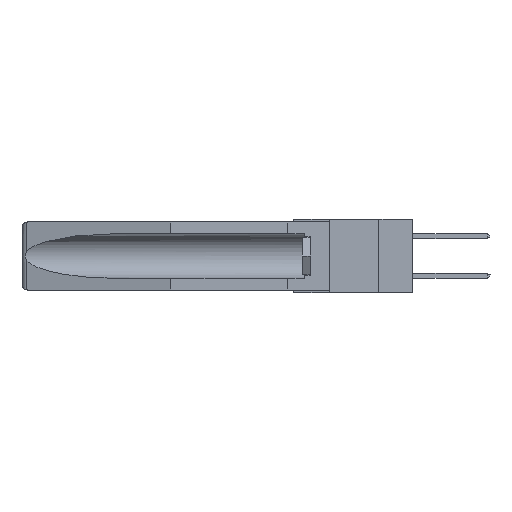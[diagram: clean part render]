
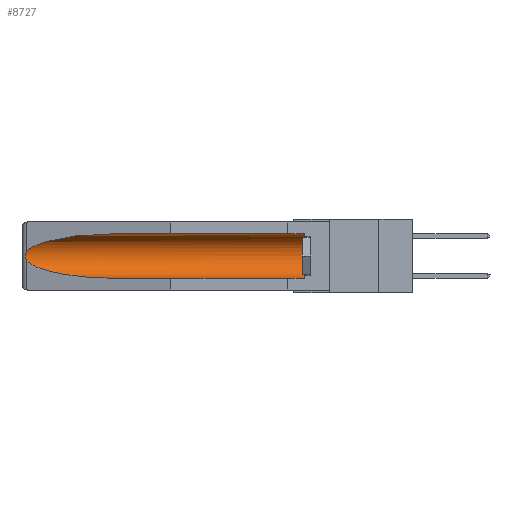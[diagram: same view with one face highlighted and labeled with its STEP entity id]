
A CAD part, left-side view. The second image highlights one B-rep face of the part: STEP entity #8727.
In plain terms, the highlighted cylindrical face has radius 2.857 mm (diameter 5.715 mm), a partial arc.
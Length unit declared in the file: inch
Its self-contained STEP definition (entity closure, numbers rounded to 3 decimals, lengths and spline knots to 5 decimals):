
#3 =( BOUNDED_CURVE ( )  B_SPLINE_CURVE ( 3, ( #23442, #5948, #15624, #5867 ),
 .UNSPECIFIED., .F., .F. ) 
 B_SPLINE_CURVE_WITH_KNOTS ( ( 4, 4 ),
 ( 0.1948, 1.5708 ),
 .UNSPECIFIED. ) 
 CURVE ( )  GEOMETRIC_REPRESENTATION_ITEM ( )  RATIONAL_B_SPLINE_CURVE ( ( 1., 0.848, 0.848, 1. ) ) 
 REPRESENTATION_ITEM ( '' )  );
#328 = EDGE_CURVE ( 'NONE', #17743, #17272, #1385, .T. ) ;
#438 = LINE ( 'NONE', #19097, #12175 ) ;
#829 = VERTEX_POINT ( 'NONE', #1903 ) ;
#1095 = ORIENTED_EDGE ( 'NONE', *, *, #6823, .T. ) ;
#1385 = B_SPLINE_CURVE_WITH_KNOTS ( 'NONE', 3,
 ( #20605, #16587, #24638, #8852, #22409, #8941, #18413, #16749, #18651, #12716 ),
 .UNSPECIFIED., .F., .F.,
 ( 4, 2, 2, 2, 4 ),
 ( 0., 0.00029, 0.00058, 0.00087, 0.00117 ),
 .UNSPECIFIED. ) ;
#1903 = CARTESIAN_POINT ( 'NONE',  ( 0.155, 0.126, -0.059 ) ) ;
#2323 = ORIENTED_EDGE ( 'NONE', *, *, #14738, .T. ) ;
#3191 = LINE ( 'NONE', #23447, #12203 ) ;
#3434 = CARTESIAN_POINT ( 'NONE',  ( 0.155, -0.30754, -0.1715 ) ) ;
#3540 = EDGE_CURVE ( 'NONE', #17736, #11007, #3191, .T. ) ;
#4085 = CARTESIAN_POINT ( 'NONE',  ( 0.155, 1.07973, -0.284 ) ) ;
#4556 = VERTEX_POINT ( 'NONE', #12770 ) ;
#4819 = CARTESIAN_POINT ( 'NONE',  ( 0.26537, 1.52718, -0.14972 ) ) ;
#4895 = CARTESIAN_POINT ( 'NONE',  ( 0.155, 1.07973, -0.059 ) ) ;
#5078 = DIRECTION ( 'NONE',  ( 0., 1., 0. ) ) ;
#5425 = DIRECTION ( 'NONE',  ( 0., -1., 0. ) ) ;
#5719 = ORIENTED_EDGE ( 'NONE', *, *, #24822, .T. ) ;
#5867 = CARTESIAN_POINT ( 'NONE',  ( 0.155, 1.07973, -0.284 ) ) ;
#5948 = CARTESIAN_POINT ( 'NONE',  ( 0.25451, 1.48313, -0.24835 ) ) ;
#6102 = CARTESIAN_POINT ( 'NONE',  ( 0.26537, 1.52718, -0.19328 ) ) ;
#6205 = FACE_OUTER_BOUND ( 'NONE', #23884, .T. ) ;
#6723 = CARTESIAN_POINT ( 'NONE',  ( 0.21114, 1.30732, -0.059 ) ) ;
#6823 = EDGE_CURVE ( 'NONE', #829, #4556, #438, .T. ) ;
#7104 = DIRECTION ( 'NONE',  ( 0., 0., 1. ) ) ;
#7859 = CARTESIAN_POINT ( 'NONE',  ( 0.26537, 1.52718, -0.14972 ) ) ;
#8727 = ADVANCED_FACE ( 'NONE', ( #6205 ), #10832, .F. ) ;
#8728 = CARTESIAN_POINT ( 'NONE',  ( 0.25451, 1.48313, -0.09465 ) ) ;
#8852 = CARTESIAN_POINT ( 'NONE',  ( 0.2673, 1.5327, -0.16383 ) ) ;
#8941 = CARTESIAN_POINT ( 'NONE',  ( 0.2675, 1.53308, -0.17534 ) ) ;
#9845 = AXIS2_PLACEMENT_3D ( 'NONE', #3434, #5078, #7104 ) ;
#10832 = CYLINDRICAL_SURFACE ( 'NONE', #9845, 0.1125 ) ;
#11007 = VERTEX_POINT ( 'NONE', #4085 ) ;
#12175 = VECTOR ( 'NONE', #13164, 39.37008 ) ;
#12203 = VECTOR ( 'NONE', #19569, 39.37008 ) ;
#12716 = CARTESIAN_POINT ( 'NONE',  ( 0.26537, 1.52718, -0.19328 ) ) ;
#12770 = CARTESIAN_POINT ( 'NONE',  ( 0.155, 1.07973, -0.059 ) ) ;
#13164 = DIRECTION ( 'NONE',  ( 0., 1., 0. ) ) ;
#13293 = DIRECTION ( 'NONE',  ( 0., 0., 1. ) ) ;
#13857 = ORIENTED_EDGE ( 'NONE', *, *, #23573, .T. ) ;
#14738 = EDGE_CURVE ( 'NONE', #17736, #829, #19754, .T. ) ;
#15480 = ORIENTED_EDGE ( 'NONE', *, *, #3540, .F. ) ;
#15624 = CARTESIAN_POINT ( 'NONE',  ( 0.21114, 1.30732, -0.284 ) ) ;
#16587 = CARTESIAN_POINT ( 'NONE',  ( 0.26597, 1.52961, -0.15275 ) ) ;
#16749 = CARTESIAN_POINT ( 'NONE',  ( 0.26655, 1.53094, -0.18657 ) ) ;
#17272 = VERTEX_POINT ( 'NONE', #6102 ) ;
#17665 = ORIENTED_EDGE ( 'NONE', *, *, #328, .T. ) ;
#17736 = VERTEX_POINT ( 'NONE', #25470 ) ;
#17743 = VERTEX_POINT ( 'NONE', #7859 ) ;
#18413 = CARTESIAN_POINT ( 'NONE',  ( 0.2673, 1.53269, -0.17917 ) ) ;
#18651 = CARTESIAN_POINT ( 'NONE',  ( 0.26597, 1.5296, -0.19026 ) ) ;
#19097 = CARTESIAN_POINT ( 'NONE',  ( 0.155, -0.30754, -0.059 ) ) ;
#19482 = AXIS2_PLACEMENT_3D ( 'NONE', #25062, #5425, #13293 ) ;
#19569 = DIRECTION ( 'NONE',  ( 0., 1., 0. ) ) ;
#19754 = CIRCLE ( 'NONE', #19482, 0.1125 ) ;
#20605 = CARTESIAN_POINT ( 'NONE',  ( 0.26537, 1.52718, -0.14972 ) ) ;
#22409 = CARTESIAN_POINT ( 'NONE',  ( 0.2675, 1.53308, -0.16763 ) ) ;
#23345 =( BOUNDED_CURVE ( )  B_SPLINE_CURVE ( 3, ( #4895, #6723, #8728, #4819 ),
 .UNSPECIFIED., .F., .F. ) 
 B_SPLINE_CURVE_WITH_KNOTS ( ( 4, 4 ),
 ( 4.71239, 6.08839 ),
 .UNSPECIFIED. ) 
 CURVE ( )  GEOMETRIC_REPRESENTATION_ITEM ( )  RATIONAL_B_SPLINE_CURVE ( ( 1., 0.848, 0.848, 1. ) ) 
 REPRESENTATION_ITEM ( '' )  );
#23442 = CARTESIAN_POINT ( 'NONE',  ( 0.26537, 1.52718, -0.19328 ) ) ;
#23447 = CARTESIAN_POINT ( 'NONE',  ( 0.155, -0.30754, -0.284 ) ) ;
#23573 = EDGE_CURVE ( 'NONE', #17272, #11007, #3, .T. ) ;
#23884 = EDGE_LOOP ( 'NONE', ( #5719, #17665, #13857, #15480, #2323, #1095 ) ) ;
#24638 = CARTESIAN_POINT ( 'NONE',  ( 0.26654, 1.53092, -0.15636 ) ) ;
#24822 = EDGE_CURVE ( 'NONE', #4556, #17743, #23345, .T. ) ;
#25062 = CARTESIAN_POINT ( 'NONE',  ( 0.155, 0.126, -0.1715 ) ) ;
#25470 = CARTESIAN_POINT ( 'NONE',  ( 0.155, 0.126, -0.284 ) ) ;
